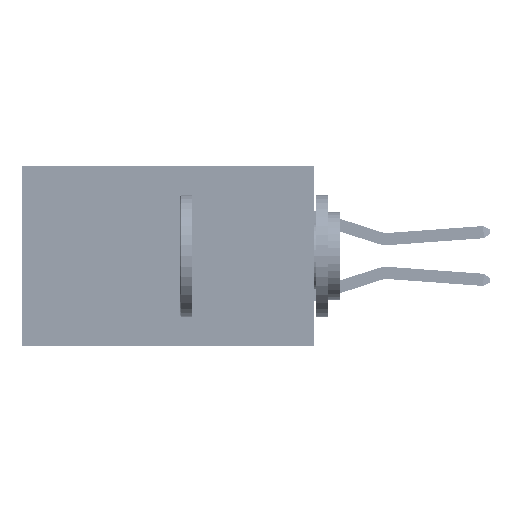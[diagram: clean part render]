
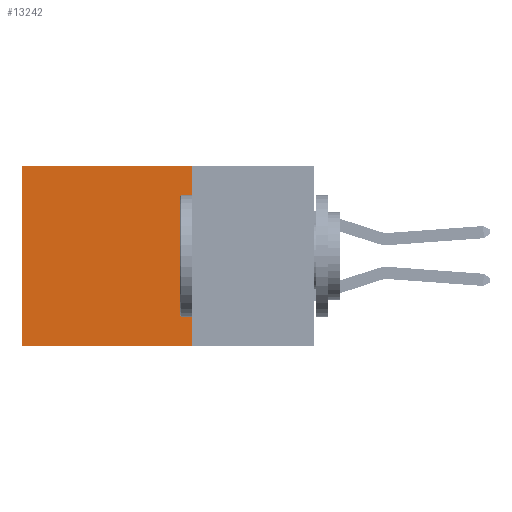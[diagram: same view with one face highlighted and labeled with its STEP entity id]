
A CAD part, left-side view. The second image highlights one B-rep face of the part: STEP entity #13242.
In plain terms, the highlighted planar face has unit normal (-1, 0, 0).
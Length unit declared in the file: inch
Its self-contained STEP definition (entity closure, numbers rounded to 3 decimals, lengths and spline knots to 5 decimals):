
#47 = PLANE ( 'NONE',  #15898 ) ;
#3943 = DIRECTION ( 'NONE',  ( 0., 1., 0. ) ) ;
#4325 = VERTEX_POINT ( 'NONE', #41969 ) ;
#4329 = LINE ( 'NONE', #4980, #36532 ) ;
#4571 = DIRECTION ( 'NONE',  ( 0., 1., 0. ) ) ;
#4980 = CARTESIAN_POINT ( 'NONE',  ( 0.2875, 0.6, 0. ) ) ;
#6423 = VERTEX_POINT ( 'NONE', #29741 ) ;
#6776 = CARTESIAN_POINT ( 'NONE',  ( 0.2875, 0.6, 0. ) ) ;
#8209 = LINE ( 'NONE', #25055, #40479 ) ;
#8682 = LINE ( 'NONE', #27822, #20907 ) ;
#11998 = VERTEX_POINT ( 'NONE', #6776 ) ;
#12564 = ORIENTED_EDGE ( 'NONE', *, *, #42627, .T. ) ;
#13242 = ADVANCED_FACE ( 'NONE', ( #42638 ), #47, .F. ) ;
#15091 = ORIENTED_EDGE ( 'NONE', *, *, #44914, .F. ) ;
#15898 = AXIS2_PLACEMENT_3D ( 'NONE', #45172, #20491, #49282 ) ;
#20491 = DIRECTION ( 'NONE',  ( 1., 0., 0. ) ) ;
#20907 = VECTOR ( 'NONE', #40278, 39.37008 ) ;
#24439 = EDGE_LOOP ( 'NONE', ( #51008, #33558, #15091, #12564 ) ) ;
#25055 = CARTESIAN_POINT ( 'NONE',  ( 0.2875, 0.25, 0. ) ) ;
#27822 = CARTESIAN_POINT ( 'NONE',  ( 0.2875, 0.25, 0. ) ) ;
#29741 = CARTESIAN_POINT ( 'NONE',  ( 0.2875, 0.6, -0.37 ) ) ;
#30906 = EDGE_CURVE ( 'NONE', #4325, #6423, #34874, .T. ) ;
#32575 = CARTESIAN_POINT ( 'NONE',  ( 0.2875, 0.25, -0.37 ) ) ;
#33558 = ORIENTED_EDGE ( 'NONE', *, *, #30906, .F. ) ;
#34874 = LINE ( 'NONE', #32575, #49571 ) ;
#36343 = CARTESIAN_POINT ( 'NONE',  ( 0.2875, 0.25, 0. ) ) ;
#36532 = VECTOR ( 'NONE', #37744, 39.37008 ) ;
#37744 = DIRECTION ( 'NONE',  ( 0., 0., -1. ) ) ;
#40278 = DIRECTION ( 'NONE',  ( 0., 0., -1. ) ) ;
#40479 = VECTOR ( 'NONE', #4571, 39.37008 ) ;
#41969 = CARTESIAN_POINT ( 'NONE',  ( 0.2875, 0.25, -0.37 ) ) ;
#42627 = EDGE_CURVE ( 'NONE', #49889, #11998, #8209, .T. ) ;
#42638 = FACE_OUTER_BOUND ( 'NONE', #24439, .T. ) ;
#43194 = EDGE_CURVE ( 'NONE', #11998, #6423, #4329, .T. ) ;
#44914 = EDGE_CURVE ( 'NONE', #49889, #4325, #8682, .T. ) ;
#45172 = CARTESIAN_POINT ( 'NONE',  ( 0.2875, 0.25, 0. ) ) ;
#49282 = DIRECTION ( 'NONE',  ( 0., 0., -1. ) ) ;
#49571 = VECTOR ( 'NONE', #3943, 39.37008 ) ;
#49889 = VERTEX_POINT ( 'NONE', #36343 ) ;
#51008 = ORIENTED_EDGE ( 'NONE', *, *, #43194, .T. ) ;
